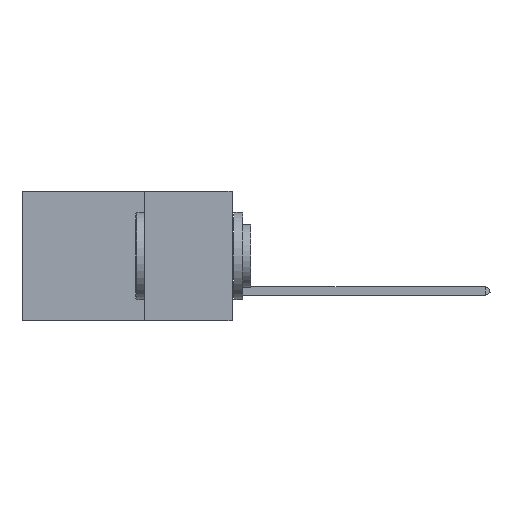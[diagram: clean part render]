
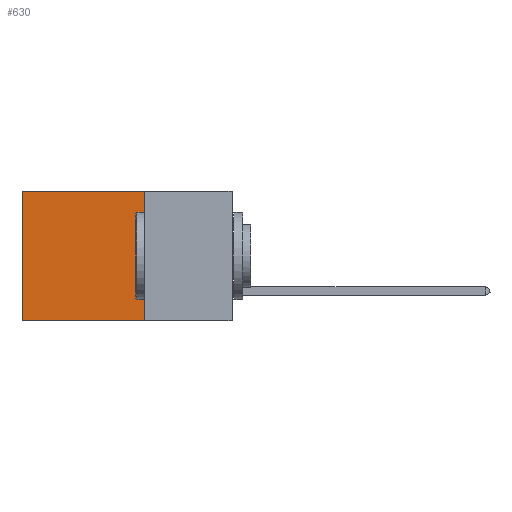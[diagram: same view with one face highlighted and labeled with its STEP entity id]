
A CAD part, left-side view. The second image highlights one B-rep face of the part: STEP entity #630.
In plain terms, the highlighted planar face has unit normal (-1, 0, 0).
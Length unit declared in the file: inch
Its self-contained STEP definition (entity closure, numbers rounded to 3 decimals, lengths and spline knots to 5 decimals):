
#49 = EDGE_CURVE ( 'NONE', #12909, #14046, #10914, .T. ) ;
#630 = ADVANCED_FACE ( 'NONE', ( #5671 ), #10946, .F. ) ;
#1393 = DIRECTION ( 'NONE',  ( 0., 0., -1. ) ) ;
#2080 = ORIENTED_EDGE ( 'NONE', *, *, #49, .T. ) ;
#2380 = CARTESIAN_POINT ( 'NONE',  ( 0.2875, 0.25, -0.37 ) ) ;
#2403 = ORIENTED_EDGE ( 'NONE', *, *, #9570, .F. ) ;
#2848 = VERTEX_POINT ( 'NONE', #13497 ) ;
#3308 = CARTESIAN_POINT ( 'NONE',  ( 0.2875, 0.25, 0. ) ) ;
#3492 = VECTOR ( 'NONE', #12061, 39.37008 ) ;
#3539 = EDGE_CURVE ( 'NONE', #9439, #2848, #15826, .T. ) ;
#3949 = DIRECTION ( 'NONE',  ( 0., 0., -1. ) ) ;
#5500 = VECTOR ( 'NONE', #3949, 39.37008 ) ;
#5671 = FACE_OUTER_BOUND ( 'NONE', #10790, .T. ) ;
#6065 = VECTOR ( 'NONE', #7195, 39.37008 ) ;
#6879 = AXIS2_PLACEMENT_3D ( 'NONE', #12620, #11223, #1393 ) ;
#7195 = DIRECTION ( 'NONE',  ( 0., 1., 0. ) ) ;
#8502 = CARTESIAN_POINT ( 'NONE',  ( 0.2875, 0.25, 0. ) ) ;
#9439 = VERTEX_POINT ( 'NONE', #3308 ) ;
#9570 = EDGE_CURVE ( 'NONE', #2848, #14046, #15361, .T. ) ;
#9792 = VECTOR ( 'NONE', #12324, 39.37008 ) ;
#10458 = EDGE_CURVE ( 'NONE', #9439, #12909, #11682, .T. ) ;
#10548 = CARTESIAN_POINT ( 'NONE',  ( 0.2875, 0.6, -0.37 ) ) ;
#10755 = CARTESIAN_POINT ( 'NONE',  ( 0.2875, 0.25, 0. ) ) ;
#10790 = EDGE_LOOP ( 'NONE', ( #2080, #2403, #15598, #13658 ) ) ;
#10914 = LINE ( 'NONE', #11294, #5500 ) ;
#10946 = PLANE ( 'NONE',  #6879 ) ;
#11223 = DIRECTION ( 'NONE',  ( 1., 0., 0. ) ) ;
#11294 = CARTESIAN_POINT ( 'NONE',  ( 0.2875, 0.6, 0. ) ) ;
#11682 = LINE ( 'NONE', #8502, #6065 ) ;
#12061 = DIRECTION ( 'NONE',  ( 0., 0., -1. ) ) ;
#12324 = DIRECTION ( 'NONE',  ( 0., 1., 0. ) ) ;
#12620 = CARTESIAN_POINT ( 'NONE',  ( 0.2875, 0.25, 0. ) ) ;
#12909 = VERTEX_POINT ( 'NONE', #12963 ) ;
#12963 = CARTESIAN_POINT ( 'NONE',  ( 0.2875, 0.6, 0. ) ) ;
#13497 = CARTESIAN_POINT ( 'NONE',  ( 0.2875, 0.25, -0.37 ) ) ;
#13658 = ORIENTED_EDGE ( 'NONE', *, *, #10458, .T. ) ;
#14046 = VERTEX_POINT ( 'NONE', #10548 ) ;
#15361 = LINE ( 'NONE', #2380, #9792 ) ;
#15598 = ORIENTED_EDGE ( 'NONE', *, *, #3539, .F. ) ;
#15826 = LINE ( 'NONE', #10755, #3492 ) ;
